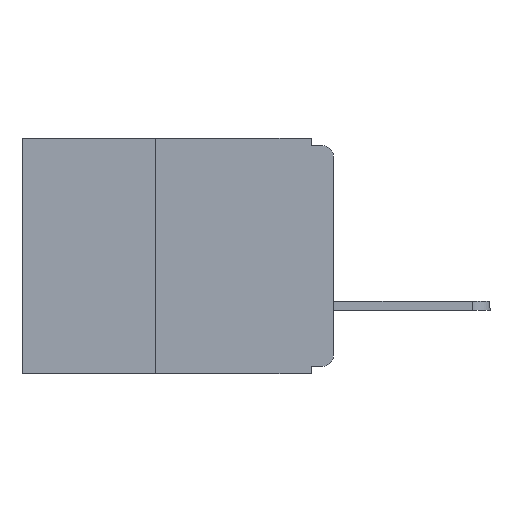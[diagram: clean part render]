
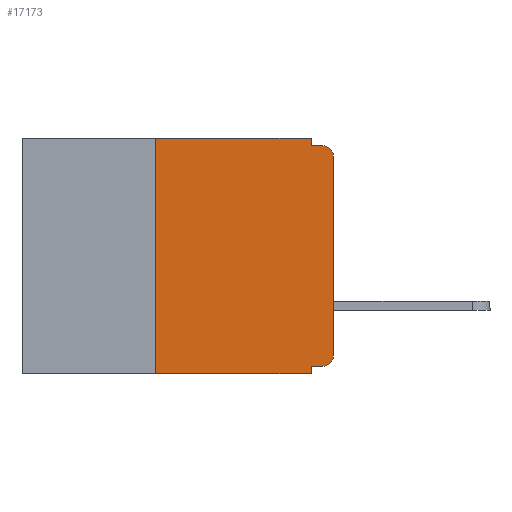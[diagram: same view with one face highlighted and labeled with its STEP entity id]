
A CAD part, left-side view. The second image highlights one B-rep face of the part: STEP entity #17173.
In plain terms, the highlighted planar face has unit normal (-1, 0, 0).
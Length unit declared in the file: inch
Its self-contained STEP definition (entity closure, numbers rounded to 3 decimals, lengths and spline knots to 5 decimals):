
#79 = LINE ( 'NONE', #20704, #9610 ) ;
#414 = EDGE_CURVE ( 'NONE', #2345, #10083, #3880, .T. ) ;
#605 = EDGE_CURVE ( 'NONE', #20321, #2345, #23661, .T. ) ;
#1079 = LINE ( 'NONE', #9984, #19419 ) ;
#1678 = CARTESIAN_POINT ( 'NONE',  ( 0., 0., -0.32 ) ) ;
#1771 = CARTESIAN_POINT ( 'NONE',  ( 0., 0.031, -0.32 ) ) ;
#2042 = CARTESIAN_POINT ( 'NONE',  ( 0., 0.031, -0.33 ) ) ;
#2327 = CARTESIAN_POINT ( 'NONE',  ( 0., 0., -0.305 ) ) ;
#2345 = VERTEX_POINT ( 'NONE', #1771 ) ;
#2684 = CARTESIAN_POINT ( 'NONE',  ( 0., 0.437, 0. ) ) ;
#2981 = DIRECTION ( 'NONE',  ( -1., 0., 0. ) ) ;
#2983 = VERTEX_POINT ( 'NONE', #16568 ) ;
#2991 = EDGE_CURVE ( 'NONE', #17843, #23306, #19494, .T. ) ;
#3194 = DIRECTION ( 'NONE',  ( -1., 0., 0. ) ) ;
#3375 = LINE ( 'NONE', #16357, #22280 ) ;
#3880 = LINE ( 'NONE', #2042, #8300 ) ;
#3925 = AXIS2_PLACEMENT_3D ( 'NONE', #14440, #3194, #16347 ) ;
#4520 = CIRCLE ( 'NONE', #3925, 0.015 ) ;
#4523 = CARTESIAN_POINT ( 'NONE',  ( 0., 0.015, -0.32 ) ) ;
#5361 = FACE_OUTER_BOUND ( 'NONE', #23155, .T. ) ;
#6037 = DIRECTION ( 'NONE',  ( 0., -1., 0. ) ) ;
#6169 = VERTEX_POINT ( 'NONE', #6507 ) ;
#6507 = CARTESIAN_POINT ( 'NONE',  ( 0., 0.25, -0.33 ) ) ;
#6599 = AXIS2_PLACEMENT_3D ( 'NONE', #14233, #2981, #16144 ) ;
#6604 = ORIENTED_EDGE ( 'NONE', *, *, #13981, .F. ) ;
#7370 = ORIENTED_EDGE ( 'NONE', *, *, #2991, .F. ) ;
#8184 = EDGE_CURVE ( 'NONE', #20321, #17707, #4520, .T. ) ;
#8300 = VECTOR ( 'NONE', #16291, 39.37008 ) ;
#8730 = ORIENTED_EDGE ( 'NONE', *, *, #18900, .F. ) ;
#9169 = EDGE_CURVE ( 'NONE', #6169, #10083, #23721, .T. ) ;
#9237 = CARTESIAN_POINT ( 'NONE',  ( 0., 0.015, -0.01 ) ) ;
#9474 = VECTOR ( 'NONE', #13685, 39.37008 ) ;
#9598 = ORIENTED_EDGE ( 'NONE', *, *, #16693, .F. ) ;
#9610 = VECTOR ( 'NONE', #18791, 39.37008 ) ;
#9984 = CARTESIAN_POINT ( 'NONE',  ( 0., 0.031, 0. ) ) ;
#10083 = VERTEX_POINT ( 'NONE', #18177 ) ;
#10303 = DIRECTION ( 'NONE',  ( 1., 0., 0. ) ) ;
#10402 = CARTESIAN_POINT ( 'NONE',  ( 0., 0.25, 0. ) ) ;
#12470 = ORIENTED_EDGE ( 'NONE', *, *, #605, .F. ) ;
#12515 = CARTESIAN_POINT ( 'NONE',  ( 0., 0.437, 0. ) ) ;
#13116 = CARTESIAN_POINT ( 'NONE',  ( 0., 0.031, 0. ) ) ;
#13213 = AXIS2_PLACEMENT_3D ( 'NONE', #2684, #10303, #23521 ) ;
#13261 = VERTEX_POINT ( 'NONE', #13116 ) ;
#13505 = CARTESIAN_POINT ( 'NONE',  ( 0., 0.437, -0.33 ) ) ;
#13641 = CARTESIAN_POINT ( 'NONE',  ( 0., 0., -0.01 ) ) ;
#13685 = DIRECTION ( 'NONE',  ( 0., -1., 0. ) ) ;
#13981 = EDGE_CURVE ( 'NONE', #6169, #18500, #79, .T. ) ;
#14233 = CARTESIAN_POINT ( 'NONE',  ( 0., 0.015, -0.025 ) ) ;
#14440 = CARTESIAN_POINT ( 'NONE',  ( 0., 0.015, -0.305 ) ) ;
#14500 = EDGE_CURVE ( 'NONE', #17707, #2983, #3375, .T. ) ;
#15738 = ORIENTED_EDGE ( 'NONE', *, *, #8184, .T. ) ;
#15916 = ORIENTED_EDGE ( 'NONE', *, *, #16633, .T. ) ;
#16144 = DIRECTION ( 'NONE',  ( 0., 0., -1. ) ) ;
#16291 = DIRECTION ( 'NONE',  ( 0., 0., -1. ) ) ;
#16347 = DIRECTION ( 'NONE',  ( 0., 0., -1. ) ) ;
#16357 = CARTESIAN_POINT ( 'NONE',  ( 0., 0., 0. ) ) ;
#16442 = DIRECTION ( 'NONE',  ( 0., 0., 1. ) ) ;
#16568 = CARTESIAN_POINT ( 'NONE',  ( 0., 0., -0.025 ) ) ;
#16570 = LINE ( 'NONE', #12515, #21030 ) ;
#16633 = EDGE_CURVE ( 'NONE', #2983, #23306, #22830, .T. ) ;
#16693 = EDGE_CURVE ( 'NONE', #18500, #13261, #16570, .T. ) ;
#17173 = ADVANCED_FACE ( 'NONE', ( #5361 ), #21611, .F. ) ;
#17435 = ORIENTED_EDGE ( 'NONE', *, *, #14500, .T. ) ;
#17707 = VERTEX_POINT ( 'NONE', #2327 ) ;
#17843 = VERTEX_POINT ( 'NONE', #19676 ) ;
#18177 = CARTESIAN_POINT ( 'NONE',  ( 0., 0.031, -0.33 ) ) ;
#18500 = VERTEX_POINT ( 'NONE', #10402 ) ;
#18580 = VECTOR ( 'NONE', #22879, 39.37008 ) ;
#18648 = VECTOR ( 'NONE', #6037, 39.37008 ) ;
#18791 = DIRECTION ( 'NONE',  ( 0., 0., 1. ) ) ;
#18900 = EDGE_CURVE ( 'NONE', #13261, #17843, #1079, .T. ) ;
#19419 = VECTOR ( 'NONE', #21370, 39.37008 ) ;
#19494 = LINE ( 'NONE', #13641, #9474 ) ;
#19676 = CARTESIAN_POINT ( 'NONE',  ( 0., 0.031, -0.01 ) ) ;
#20321 = VERTEX_POINT ( 'NONE', #4523 ) ;
#20704 = CARTESIAN_POINT ( 'NONE',  ( 0., 0.25, -0.33 ) ) ;
#21030 = VECTOR ( 'NONE', #23879, 39.37008 ) ;
#21370 = DIRECTION ( 'NONE',  ( 0., 0., -1. ) ) ;
#21611 = PLANE ( 'NONE',  #13213 ) ;
#22280 = VECTOR ( 'NONE', #16442, 39.37008 ) ;
#22830 = CIRCLE ( 'NONE', #6599, 0.015 ) ;
#22879 = DIRECTION ( 'NONE',  ( 0., 1., 0. ) ) ;
#23155 = EDGE_LOOP ( 'NONE', ( #17435, #15916, #7370, #8730, #9598, #6604, #23646, #24471, #12470, #15738 ) ) ;
#23306 = VERTEX_POINT ( 'NONE', #9237 ) ;
#23521 = DIRECTION ( 'NONE',  ( 0., 0., -1. ) ) ;
#23646 = ORIENTED_EDGE ( 'NONE', *, *, #9169, .T. ) ;
#23661 = LINE ( 'NONE', #1678, #18580 ) ;
#23721 = LINE ( 'NONE', #13505, #18648 ) ;
#23879 = DIRECTION ( 'NONE',  ( 0., -1., 0. ) ) ;
#24471 = ORIENTED_EDGE ( 'NONE', *, *, #414, .F. ) ;
